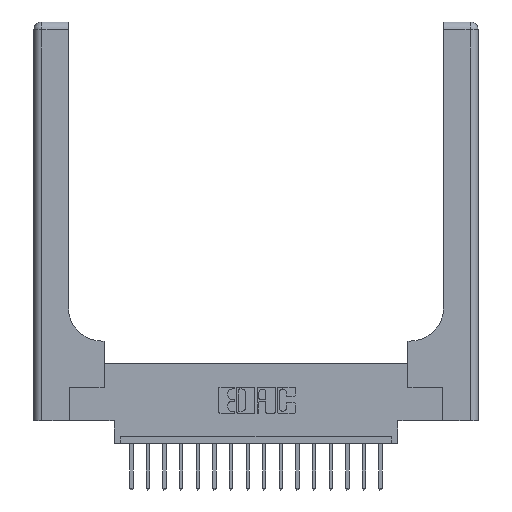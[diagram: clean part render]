
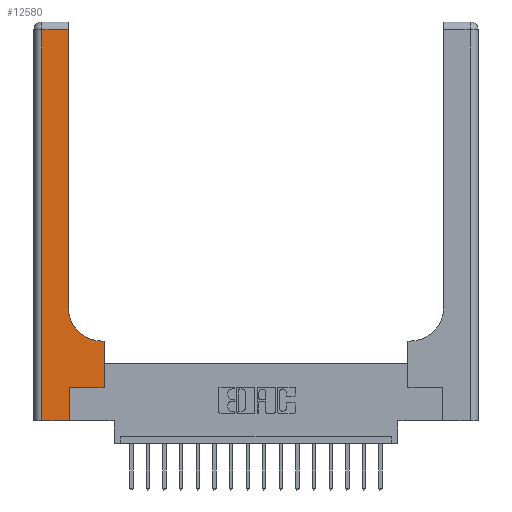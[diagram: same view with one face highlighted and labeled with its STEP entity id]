
A CAD part, top view. The second image highlights one B-rep face of the part: STEP entity #12580.
In plain terms, the highlighted planar face has unit normal (0, 0, 1).
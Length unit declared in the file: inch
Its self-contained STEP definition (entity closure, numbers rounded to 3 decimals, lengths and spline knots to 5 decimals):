
#232 = EDGE_CURVE ( 'NONE', #6255, #13595, #2332, .T. ) ;
#959 = LINE ( 'NONE', #19006, #13593 ) ;
#1048 = VECTOR ( 'NONE', #10350, 39.37008 ) ;
#1152 = CARTESIAN_POINT ( 'NONE',  ( 0., 2.94, 0.37 ) ) ;
#1437 = ORIENTED_EDGE ( 'NONE', *, *, #8292, .T. ) ;
#1479 = EDGE_CURVE ( 'NONE', #11418, #6594, #959, .T. ) ;
#2123 = DIRECTION ( 'NONE',  ( 1., 0., 0. ) ) ;
#2332 = CIRCLE ( 'NONE', #5729, 0.25 ) ;
#2595 = VERTEX_POINT ( 'NONE', #13316 ) ;
#2652 = EDGE_CURVE ( 'NONE', #13640, #16423, #17268, .T. ) ;
#2687 = CARTESIAN_POINT ( 'NONE',  ( 0.51, 0.85, 0.37 ) ) ;
#3036 = VERTEX_POINT ( 'NONE', #15085 ) ;
#3196 = FACE_OUTER_BOUND ( 'NONE', #13835, .T. ) ;
#3333 = ORIENTED_EDGE ( 'NONE', *, *, #9883, .T. ) ;
#3546 = VECTOR ( 'NONE', #13201, 39.37008 ) ;
#3932 = DIRECTION ( 'NONE',  ( -1., 0., 0. ) ) ;
#3944 = EDGE_CURVE ( 'NONE', #9135, #3036, #6703, .T. ) ;
#4378 = EDGE_CURVE ( 'NONE', #6594, #6255, #6866, .T. ) ;
#4980 = VECTOR ( 'NONE', #9169, 39.37008 ) ;
#5600 = ORIENTED_EDGE ( 'NONE', *, *, #10465, .T. ) ;
#5729 = AXIS2_PLACEMENT_3D ( 'NONE', #2687, #9716, #11447 ) ;
#6051 = LINE ( 'NONE', #16244, #4980 ) ;
#6255 = VERTEX_POINT ( 'NONE', #15538 ) ;
#6299 = VECTOR ( 'NONE', #15533, 39.37008 ) ;
#6388 = CARTESIAN_POINT ( 'NONE',  ( 0.06, 0., 0.37 ) ) ;
#6594 = VERTEX_POINT ( 'NONE', #18608 ) ;
#6703 = LINE ( 'NONE', #11056, #13709 ) ;
#6866 = LINE ( 'NONE', #12409, #7878 ) ;
#7623 = CARTESIAN_POINT ( 'NONE',  ( 0.265, 0.25, 0.37 ) ) ;
#7878 = VECTOR ( 'NONE', #3932, 39.37008 ) ;
#8292 = EDGE_CURVE ( 'NONE', #13595, #13640, #6051, .T. ) ;
#8853 = DIRECTION ( 'NONE',  ( -1., 0., 0. ) ) ;
#9135 = VERTEX_POINT ( 'NONE', #6388 ) ;
#9138 = DIRECTION ( 'NONE',  ( 0., 0., -1. ) ) ;
#9169 = DIRECTION ( 'NONE',  ( 0., 1., 0. ) ) ;
#9242 = AXIS2_PLACEMENT_3D ( 'NONE', #10301, #9138, #8853 ) ;
#9440 = CARTESIAN_POINT ( 'NONE',  ( 0.06, 3., 0.37 ) ) ;
#9489 = ORIENTED_EDGE ( 'NONE', *, *, #1479, .T. ) ;
#9644 = EDGE_CURVE ( 'NONE', #3036, #2595, #16502, .T. ) ;
#9716 = DIRECTION ( 'NONE',  ( 0., 0., -1. ) ) ;
#9883 = EDGE_CURVE ( 'NONE', #16423, #9135, #18050, .T. ) ;
#10209 = CARTESIAN_POINT ( 'NONE',  ( 0.26, 0.85, 0.37 ) ) ;
#10301 = CARTESIAN_POINT ( 'NONE',  ( 0., 3., 0.37 ) ) ;
#10350 = DIRECTION ( 'NONE',  ( 1., 0., 0. ) ) ;
#10465 = EDGE_CURVE ( 'NONE', #2595, #11418, #17892, .T. ) ;
#10684 = CARTESIAN_POINT ( 'NONE',  ( 0.06, 2.94, 0.37 ) ) ;
#11056 = CARTESIAN_POINT ( 'NONE',  ( 0., 0., 0.37 ) ) ;
#11098 = ORIENTED_EDGE ( 'NONE', *, *, #2652, .T. ) ;
#11210 = ORIENTED_EDGE ( 'NONE', *, *, #4378, .T. ) ;
#11418 = VERTEX_POINT ( 'NONE', #12516 ) ;
#11447 = DIRECTION ( 'NONE',  ( 1., 0., 0. ) ) ;
#11868 = DIRECTION ( 'NONE',  ( 0., 1., 0. ) ) ;
#12409 = CARTESIAN_POINT ( 'NONE',  ( 0.26, 0.6, 0.37 ) ) ;
#12467 = ORIENTED_EDGE ( 'NONE', *, *, #232, .T. ) ;
#12516 = CARTESIAN_POINT ( 'NONE',  ( 0.528, 0.25, 0.37 ) ) ;
#12580 = ADVANCED_FACE ( 'NONE', ( #3196 ), #16489, .F. ) ;
#12758 = CARTESIAN_POINT ( 'NONE',  ( 0.26, 2.94, 0.37 ) ) ;
#13201 = DIRECTION ( 'NONE',  ( -1., 0., 0. ) ) ;
#13316 = CARTESIAN_POINT ( 'NONE',  ( 0.265, 0.25, 0.37 ) ) ;
#13320 = CARTESIAN_POINT ( 'NONE',  ( 0.265, 0., 0.37 ) ) ;
#13593 = VECTOR ( 'NONE', #14166, 39.37008 ) ;
#13595 = VERTEX_POINT ( 'NONE', #10209 ) ;
#13640 = VERTEX_POINT ( 'NONE', #12758 ) ;
#13709 = VECTOR ( 'NONE', #2123, 39.37008 ) ;
#13835 = EDGE_LOOP ( 'NONE', ( #1437, #11098, #3333, #18227, #19053, #5600, #9489, #11210, #12467 ) ) ;
#14166 = DIRECTION ( 'NONE',  ( 0., 1., 0. ) ) ;
#15085 = CARTESIAN_POINT ( 'NONE',  ( 0.265, 0., 0.37 ) ) ;
#15533 = DIRECTION ( 'NONE',  ( 0., -1., 0. ) ) ;
#15538 = CARTESIAN_POINT ( 'NONE',  ( 0.51, 0.6, 0.37 ) ) ;
#16244 = CARTESIAN_POINT ( 'NONE',  ( 0.26, 3., 0.37 ) ) ;
#16423 = VERTEX_POINT ( 'NONE', #10684 ) ;
#16489 = PLANE ( 'NONE',  #9242 ) ;
#16502 = LINE ( 'NONE', #13320, #18121 ) ;
#17268 = LINE ( 'NONE', #1152, #3546 ) ;
#17892 = LINE ( 'NONE', #7623, #1048 ) ;
#18050 = LINE ( 'NONE', #9440, #6299 ) ;
#18121 = VECTOR ( 'NONE', #11868, 39.37008 ) ;
#18227 = ORIENTED_EDGE ( 'NONE', *, *, #3944, .T. ) ;
#18608 = CARTESIAN_POINT ( 'NONE',  ( 0.528, 0.6, 0.37 ) ) ;
#19006 = CARTESIAN_POINT ( 'NONE',  ( 0.528, 0.25, 0.37 ) ) ;
#19053 = ORIENTED_EDGE ( 'NONE', *, *, #9644, .T. ) ;
